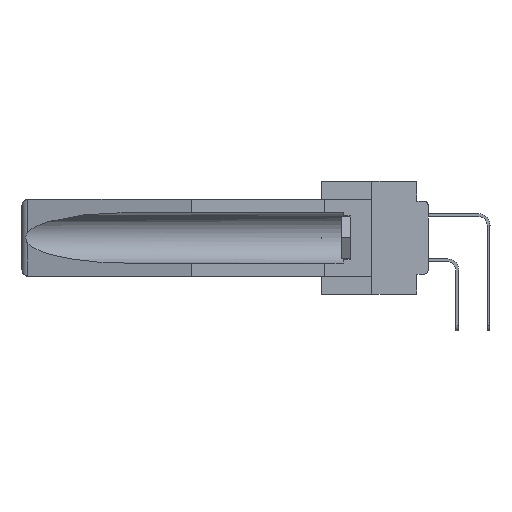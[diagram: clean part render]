
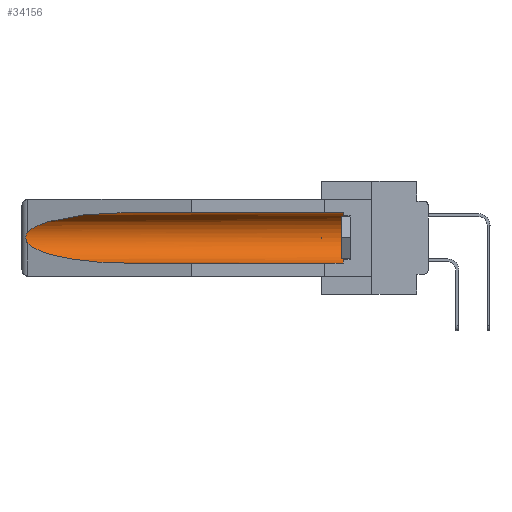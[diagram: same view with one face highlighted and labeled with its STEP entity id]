
A CAD part, left-side view. The second image highlights one B-rep face of the part: STEP entity #34156.
In plain terms, the highlighted cylindrical face has radius 2.857 mm (diameter 5.715 mm), a partial arc.
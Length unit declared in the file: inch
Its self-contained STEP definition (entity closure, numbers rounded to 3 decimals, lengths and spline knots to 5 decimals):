
#579 = CARTESIAN_POINT ( 'NONE',  ( 0.26597, 1.52961, -0.15275 ) ) ;
#1005 = VECTOR ( 'NONE', #34387, 39.37008 ) ;
#2394 = VERTEX_POINT ( 'NONE', #6774 ) ;
#3212 = VERTEX_POINT ( 'NONE', #18427 ) ;
#3299 = CARTESIAN_POINT ( 'NONE',  ( 0.26654, 1.53092, -0.15636 ) ) ;
#3692 = CARTESIAN_POINT ( 'NONE',  ( 0.155, -0.30754, -0.1715 ) ) ;
#3702 = CARTESIAN_POINT ( 'NONE',  ( 0.26597, 1.5296, -0.19026 ) ) ;
#4014 = EDGE_LOOP ( 'NONE', ( #10649, #23673, #29621, #22232, #26493, #22862 ) ) ;
#4562 = B_SPLINE_CURVE_WITH_KNOTS ( 'NONE', 3,
 ( #23132, #579, #3299, #16031, #35639, #32295, #35027, #26055, #3702, #16226 ),
 .UNSPECIFIED., .F., .F.,
 ( 4, 2, 2, 2, 4 ),
 ( 0., 0.00029, 0.00058, 0.00087, 0.00117 ),
 .UNSPECIFIED. ) ;
#5340 = EDGE_CURVE ( 'NONE', #3212, #17020, #26851, .T. ) ;
#6761 = DIRECTION ( 'NONE',  ( 0., 0., 1. ) ) ;
#6774 = CARTESIAN_POINT ( 'NONE',  ( 0.155, 1.07973, -0.284 ) ) ;
#8168 = VERTEX_POINT ( 'NONE', #28020 ) ;
#10649 = ORIENTED_EDGE ( 'NONE', *, *, #32266, .T. ) ;
#10782 =( BOUNDED_CURVE ( )  B_SPLINE_CURVE ( 3, ( #23128, #16634, #19977, #29353 ),
 .UNSPECIFIED., .F., .F. ) 
 B_SPLINE_CURVE_WITH_KNOTS ( ( 4, 4 ),
 ( 4.71239, 6.08839 ),
 .UNSPECIFIED. ) 
 CURVE ( )  GEOMETRIC_REPRESENTATION_ITEM ( )  RATIONAL_B_SPLINE_CURVE ( ( 1., 0.848, 0.848, 1. ) ) 
 REPRESENTATION_ITEM ( '' )  );
#10982 = CARTESIAN_POINT ( 'NONE',  ( 0.155, -0.30754, -0.059 ) ) ;
#12593 = EDGE_CURVE ( 'NONE', #18725, #3212, #21797, .T. ) ;
#12940 = AXIS2_PLACEMENT_3D ( 'NONE', #3692, #35018, #29149 ) ;
#14955 = CARTESIAN_POINT ( 'NONE',  ( 0.155, 0.126, -0.284 ) ) ;
#15065 =( BOUNDED_CURVE ( )  B_SPLINE_CURVE ( 3, ( #32140, #29012, #35486, #32355 ),
 .UNSPECIFIED., .F., .F. ) 
 B_SPLINE_CURVE_WITH_KNOTS ( ( 4, 4 ),
 ( 0.1948, 1.5708 ),
 .UNSPECIFIED. ) 
 CURVE ( )  GEOMETRIC_REPRESENTATION_ITEM ( )  RATIONAL_B_SPLINE_CURVE ( ( 1., 0.848, 0.848, 1. ) ) 
 REPRESENTATION_ITEM ( '' )  );
#15984 = CARTESIAN_POINT ( 'NONE',  ( 0.155, 0.126, -0.1715 ) ) ;
#16031 = CARTESIAN_POINT ( 'NONE',  ( 0.2673, 1.5327, -0.16383 ) ) ;
#16226 = CARTESIAN_POINT ( 'NONE',  ( 0.26537, 1.52718, -0.19328 ) ) ;
#16634 = CARTESIAN_POINT ( 'NONE',  ( 0.21114, 1.30732, -0.059 ) ) ;
#17020 = VERTEX_POINT ( 'NONE', #27953 ) ;
#18427 = CARTESIAN_POINT ( 'NONE',  ( 0.155, 0.126, -0.059 ) ) ;
#18725 = VERTEX_POINT ( 'NONE', #14955 ) ;
#19977 = CARTESIAN_POINT ( 'NONE',  ( 0.25451, 1.48313, -0.09465 ) ) ;
#21451 = LINE ( 'NONE', #34169, #1005 ) ;
#21797 = CIRCLE ( 'NONE', #30423, 0.1125 ) ;
#21799 = CARTESIAN_POINT ( 'NONE',  ( 0.26537, 1.52718, -0.14972 ) ) ;
#22232 = ORIENTED_EDGE ( 'NONE', *, *, #22907, .F. ) ;
#22294 = FACE_OUTER_BOUND ( 'NONE', #4014, .T. ) ;
#22862 = ORIENTED_EDGE ( 'NONE', *, *, #5340, .T. ) ;
#22907 = EDGE_CURVE ( 'NONE', #18725, #2394, #21451, .T. ) ;
#23128 = CARTESIAN_POINT ( 'NONE',  ( 0.155, 1.07973, -0.059 ) ) ;
#23132 = CARTESIAN_POINT ( 'NONE',  ( 0.26537, 1.52718, -0.14972 ) ) ;
#23673 = ORIENTED_EDGE ( 'NONE', *, *, #40159, .T. ) ;
#26055 = CARTESIAN_POINT ( 'NONE',  ( 0.26655, 1.53094, -0.18657 ) ) ;
#26414 = VECTOR ( 'NONE', #36455, 39.37008 ) ;
#26493 = ORIENTED_EDGE ( 'NONE', *, *, #12593, .T. ) ;
#26851 = LINE ( 'NONE', #10982, #26414 ) ;
#27953 = CARTESIAN_POINT ( 'NONE',  ( 0.155, 1.07973, -0.059 ) ) ;
#28020 = CARTESIAN_POINT ( 'NONE',  ( 0.26537, 1.52718, -0.19328 ) ) ;
#28098 = DIRECTION ( 'NONE',  ( 0., -1., 0. ) ) ;
#29012 = CARTESIAN_POINT ( 'NONE',  ( 0.25451, 1.48313, -0.24835 ) ) ;
#29149 = DIRECTION ( 'NONE',  ( 0., 0., 1. ) ) ;
#29353 = CARTESIAN_POINT ( 'NONE',  ( 0.26537, 1.52718, -0.14972 ) ) ;
#29621 = ORIENTED_EDGE ( 'NONE', *, *, #41111, .T. ) ;
#30423 = AXIS2_PLACEMENT_3D ( 'NONE', #15984, #28098, #6761 ) ;
#31096 = VERTEX_POINT ( 'NONE', #21799 ) ;
#32140 = CARTESIAN_POINT ( 'NONE',  ( 0.26537, 1.52718, -0.19328 ) ) ;
#32266 = EDGE_CURVE ( 'NONE', #17020, #31096, #10782, .T. ) ;
#32295 = CARTESIAN_POINT ( 'NONE',  ( 0.2675, 1.53308, -0.17534 ) ) ;
#32355 = CARTESIAN_POINT ( 'NONE',  ( 0.155, 1.07973, -0.284 ) ) ;
#34156 = ADVANCED_FACE ( 'NONE', ( #22294 ), #38989, .F. ) ;
#34169 = CARTESIAN_POINT ( 'NONE',  ( 0.155, -0.30754, -0.284 ) ) ;
#34387 = DIRECTION ( 'NONE',  ( 0., 1., 0. ) ) ;
#35018 = DIRECTION ( 'NONE',  ( 0., 1., 0. ) ) ;
#35027 = CARTESIAN_POINT ( 'NONE',  ( 0.2673, 1.53269, -0.17917 ) ) ;
#35486 = CARTESIAN_POINT ( 'NONE',  ( 0.21114, 1.30732, -0.284 ) ) ;
#35639 = CARTESIAN_POINT ( 'NONE',  ( 0.2675, 1.53308, -0.16763 ) ) ;
#36455 = DIRECTION ( 'NONE',  ( 0., 1., 0. ) ) ;
#38989 = CYLINDRICAL_SURFACE ( 'NONE', #12940, 0.1125 ) ;
#40159 = EDGE_CURVE ( 'NONE', #31096, #8168, #4562, .T. ) ;
#41111 = EDGE_CURVE ( 'NONE', #8168, #2394, #15065, .T. ) ;
